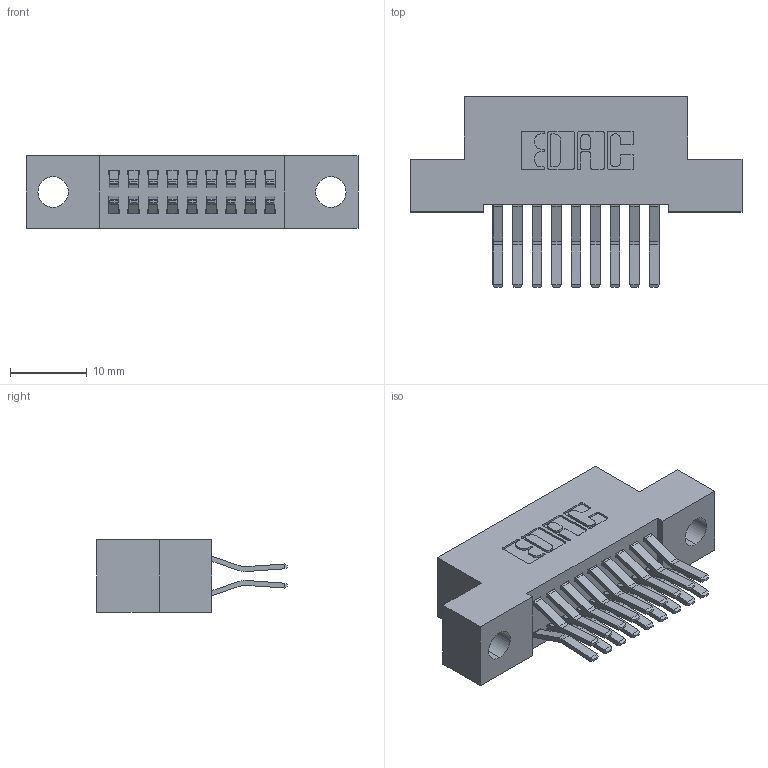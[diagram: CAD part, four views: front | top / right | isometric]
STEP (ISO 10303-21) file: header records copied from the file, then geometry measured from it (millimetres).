
FILE_DESCRIPTION (( 'STEP AP203' ), '1' );
FILE_NAME ('342-018-560-204.STEP', '2018-08-10T21:58:07', ( '' ), ( '' ), 'SwSTEP 2.0', 'SolidWorks 2016', '' );
FILE_SCHEMA (( 'CONFIG_CONTROL_DESIGN' ));
Length unit declared in the file: inch
Products named in the file (3): 342-018-560-204; 342 Part_.156 TH; 345-292-001_560 Tail
Assembly tree (19 placements, depth 2):
  342-018-560-204
    342 Part_.156 TH
    345-292-001_560 Tail  x18
Bounding box: 43.18 x 24.78 x 9.4 mm (x, y, z)
Volume: 3754.7 mm3; surface area: 5406.1 mm2
Topology: 19 solids, 19 shells, 1082 faces, 3197 edges, 2106 vertices
Faces by surface type: plane 714, cylinder 368
Entity records: 10017 total; most frequent: CARTESIAN_POINT 1698, ORIENTED_EDGE 1634, DIRECTION 1513, EDGE_CURVE 817, LINE 685, VECTOR 685, VERTEX_POINT 542, AXIS2_PLACEMENT_3D 414
